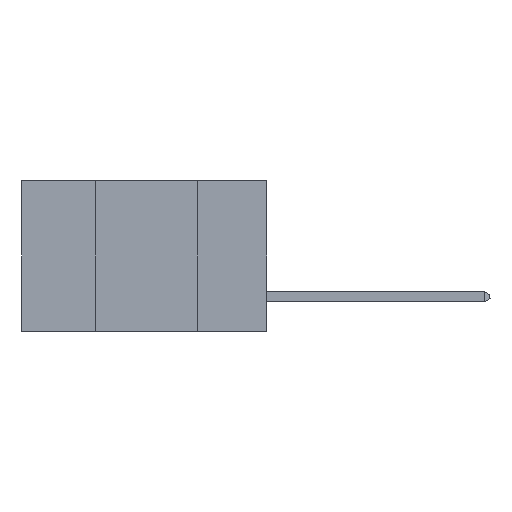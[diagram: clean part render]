
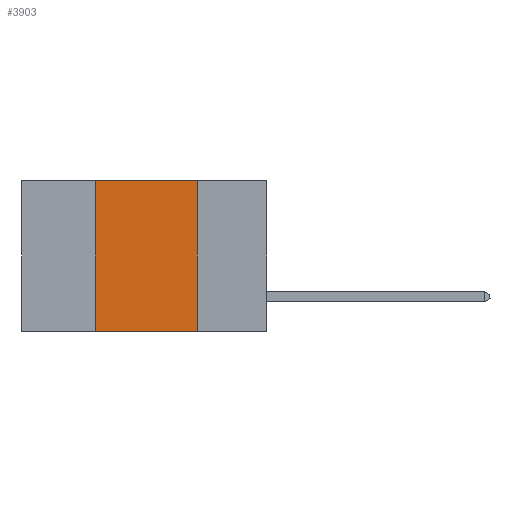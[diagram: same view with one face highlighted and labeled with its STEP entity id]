
A CAD part, left-side view. The second image highlights one B-rep face of the part: STEP entity #3903.
In plain terms, the highlighted planar face has unit normal (-1, 0, 0).
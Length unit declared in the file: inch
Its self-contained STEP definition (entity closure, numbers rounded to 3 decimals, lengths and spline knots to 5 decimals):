
#751 = AXIS2_PLACEMENT_3D ( 'NONE', #28533, #14608, #28704 ) ;
#1118 = LINE ( 'NONE', #44736, #9842 ) ;
#3903 = ADVANCED_FACE ( 'NONE', ( #25871 ), #3930, .F. ) ;
#3930 = PLANE ( 'NONE',  #751 ) ;
#4069 = VERTEX_POINT ( 'NONE', #21565 ) ;
#4173 = DIRECTION ( 'NONE',  ( 0., 0., -1. ) ) ;
#4828 = VERTEX_POINT ( 'NONE', #43049 ) ;
#6948 = EDGE_CURVE ( 'NONE', #4828, #12019, #24972, .T. ) ;
#9842 = VECTOR ( 'NONE', #37368, 39.37008 ) ;
#11180 = DIRECTION ( 'NONE',  ( 0., -1., 0. ) ) ;
#11796 = EDGE_LOOP ( 'NONE', ( #43911, #44820, #30762, #33989 ) ) ;
#12019 = VERTEX_POINT ( 'NONE', #37215 ) ;
#13479 = CARTESIAN_POINT ( 'NONE',  ( 0., 0.42, 0. ) ) ;
#13904 = LINE ( 'NONE', #29081, #39113 ) ;
#14608 = DIRECTION ( 'NONE',  ( 1., 0., 0. ) ) ;
#18931 = VECTOR ( 'NONE', #11180, 39.37008 ) ;
#21565 = CARTESIAN_POINT ( 'NONE',  ( 0., 0.17, -0.37 ) ) ;
#24631 = VERTEX_POINT ( 'NONE', #28018 ) ;
#24972 = LINE ( 'NONE', #28626, #18931 ) ;
#25871 = FACE_OUTER_BOUND ( 'NONE', #11796, .T. ) ;
#26199 = EDGE_CURVE ( 'NONE', #24631, #4828, #40294, .T. ) ;
#27541 = DIRECTION ( 'NONE',  ( 0., 0., 1. ) ) ;
#28018 = CARTESIAN_POINT ( 'NONE',  ( 0., 0.42, -0.37 ) ) ;
#28533 = CARTESIAN_POINT ( 'NONE',  ( 0., 0.6, 0. ) ) ;
#28626 = CARTESIAN_POINT ( 'NONE',  ( 0., 0.6, 0. ) ) ;
#28704 = DIRECTION ( 'NONE',  ( 0., 0., -1. ) ) ;
#29081 = CARTESIAN_POINT ( 'NONE',  ( 0., 0.17, 0. ) ) ;
#30762 = ORIENTED_EDGE ( 'NONE', *, *, #26199, .F. ) ;
#33989 = ORIENTED_EDGE ( 'NONE', *, *, #34255, .T. ) ;
#34255 = EDGE_CURVE ( 'NONE', #24631, #4069, #1118, .T. ) ;
#37215 = CARTESIAN_POINT ( 'NONE',  ( 0., 0.17, 0. ) ) ;
#37368 = DIRECTION ( 'NONE',  ( 0., -1., 0. ) ) ;
#39113 = VECTOR ( 'NONE', #4173, 39.37008 ) ;
#40294 = LINE ( 'NONE', #13479, #43017 ) ;
#43017 = VECTOR ( 'NONE', #27541, 39.37008 ) ;
#43049 = CARTESIAN_POINT ( 'NONE',  ( 0., 0.42, 0. ) ) ;
#43911 = ORIENTED_EDGE ( 'NONE', *, *, #44946, .F. ) ;
#44736 = CARTESIAN_POINT ( 'NONE',  ( 0., 0.6, -0.37 ) ) ;
#44820 = ORIENTED_EDGE ( 'NONE', *, *, #6948, .F. ) ;
#44946 = EDGE_CURVE ( 'NONE', #12019, #4069, #13904, .T. ) ;
